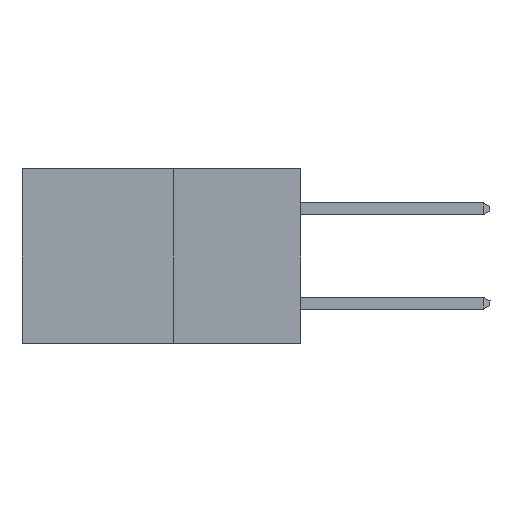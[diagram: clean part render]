
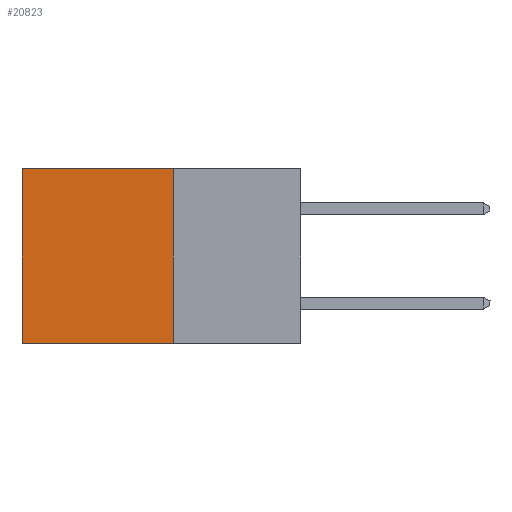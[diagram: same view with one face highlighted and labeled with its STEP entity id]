
A CAD part, left-side view. The second image highlights one B-rep face of the part: STEP entity #20823.
In plain terms, the highlighted planar face has unit normal (-1, 0, 0).
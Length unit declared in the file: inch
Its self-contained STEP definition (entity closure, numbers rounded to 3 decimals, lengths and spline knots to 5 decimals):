
#323 = EDGE_LOOP ( 'NONE', ( #4836, #20190, #9121, #21020 ) ) ;
#1153 = VERTEX_POINT ( 'NONE', #23482 ) ;
#2244 = LINE ( 'NONE', #2643, #7354 ) ;
#2643 = CARTESIAN_POINT ( 'NONE',  ( 0.277, 0.27, -0.37 ) ) ;
#3174 = VECTOR ( 'NONE', #7707, 39.37008 ) ;
#3719 = CARTESIAN_POINT ( 'NONE',  ( 0.277, 0.27, 0. ) ) ;
#4836 = ORIENTED_EDGE ( 'NONE', *, *, #15171, .T. ) ;
#7354 = VECTOR ( 'NONE', #19964, 39.37008 ) ;
#7582 = VERTEX_POINT ( 'NONE', #21204 ) ;
#7591 = CARTESIAN_POINT ( 'NONE',  ( 0.277, 0.27, -0.37 ) ) ;
#7707 = DIRECTION ( 'NONE',  ( 0., 0., -1. ) ) ;
#8908 = LINE ( 'NONE', #27016, #3174 ) ;
#9121 = ORIENTED_EDGE ( 'NONE', *, *, #21141, .F. ) ;
#12497 = CARTESIAN_POINT ( 'NONE',  ( 0.277, 0.27, -0.37 ) ) ;
#13447 = DIRECTION ( 'NONE',  ( 0., 1., 0. ) ) ;
#14706 = DIRECTION ( 'NONE',  ( 0., 0., -1. ) ) ;
#15171 = EDGE_CURVE ( 'NONE', #1153, #19650, #8908, .T. ) ;
#16202 = FACE_OUTER_BOUND ( 'NONE', #323, .T. ) ;
#16747 = PLANE ( 'NONE',  #21399 ) ;
#17560 = CARTESIAN_POINT ( 'NONE',  ( 0.277, 0.59, -0.37 ) ) ;
#18215 = VECTOR ( 'NONE', #20986, 39.37008 ) ;
#19650 = VERTEX_POINT ( 'NONE', #17560 ) ;
#19730 = EDGE_CURVE ( 'NONE', #20627, #19650, #22967, .T. ) ;
#19932 = CARTESIAN_POINT ( 'NONE',  ( 0.277, 0.27, -0.37 ) ) ;
#19964 = DIRECTION ( 'NONE',  ( 0., 0., -1. ) ) ;
#20190 = ORIENTED_EDGE ( 'NONE', *, *, #19730, .F. ) ;
#20627 = VERTEX_POINT ( 'NONE', #7591 ) ;
#20761 = EDGE_CURVE ( 'NONE', #7582, #1153, #23235, .T. ) ;
#20823 = ADVANCED_FACE ( 'NONE', ( #16202 ), #16747, .F. ) ;
#20986 = DIRECTION ( 'NONE',  ( 0., 1., 0. ) ) ;
#21020 = ORIENTED_EDGE ( 'NONE', *, *, #20761, .T. ) ;
#21141 = EDGE_CURVE ( 'NONE', #7582, #20627, #2244, .T. ) ;
#21204 = CARTESIAN_POINT ( 'NONE',  ( 0.277, 0.27, 0. ) ) ;
#21399 = AXIS2_PLACEMENT_3D ( 'NONE', #12497, #27518, #14706 ) ;
#22967 = LINE ( 'NONE', #19932, #27944 ) ;
#23235 = LINE ( 'NONE', #3719, #18215 ) ;
#23482 = CARTESIAN_POINT ( 'NONE',  ( 0.277, 0.59, 0. ) ) ;
#27016 = CARTESIAN_POINT ( 'NONE',  ( 0.277, 0.59, -0.37 ) ) ;
#27518 = DIRECTION ( 'NONE',  ( 1., 0., 0. ) ) ;
#27944 = VECTOR ( 'NONE', #13447, 39.37008 ) ;
